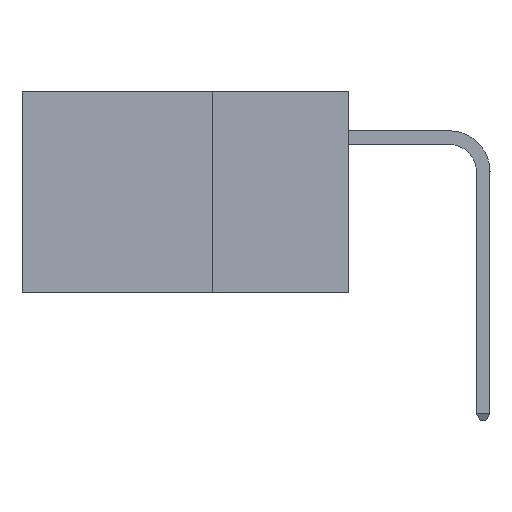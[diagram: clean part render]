
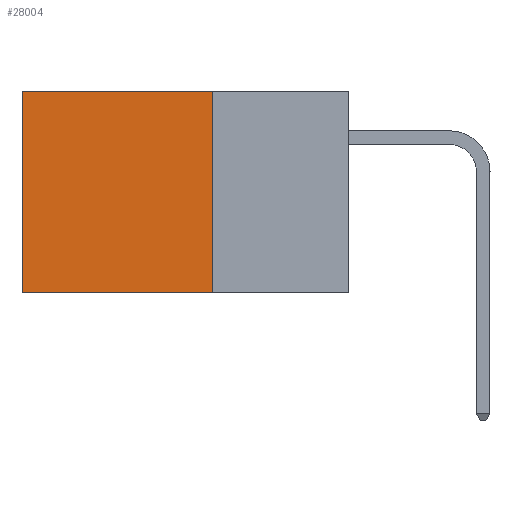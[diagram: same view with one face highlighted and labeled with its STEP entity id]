
A CAD part, left-side view. The second image highlights one B-rep face of the part: STEP entity #28004.
In plain terms, the highlighted planar face has unit normal (-1, 0, 0).
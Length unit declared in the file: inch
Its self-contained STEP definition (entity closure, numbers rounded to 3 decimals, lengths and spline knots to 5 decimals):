
#603 = ORIENTED_EDGE ( 'NONE', *, *, #15684, .F. ) ;
#860 = VERTEX_POINT ( 'NONE', #35887 ) ;
#2927 = LINE ( 'NONE', #18201, #37052 ) ;
#5528 = ORIENTED_EDGE ( 'NONE', *, *, #20811, .F. ) ;
#6387 = CARTESIAN_POINT ( 'NONE',  ( 0.2875, 0.25, 0. ) ) ;
#8119 = DIRECTION ( 'NONE',  ( 0., 1., 0. ) ) ;
#9584 = DIRECTION ( 'NONE',  ( 1., 0., 0. ) ) ;
#12715 = VERTEX_POINT ( 'NONE', #15642 ) ;
#13470 = VECTOR ( 'NONE', #40468, 39.37008 ) ;
#15327 = VERTEX_POINT ( 'NONE', #19901 ) ;
#15642 = CARTESIAN_POINT ( 'NONE',  ( 0.2875, 0.25, -0.37 ) ) ;
#15684 = EDGE_CURVE ( 'NONE', #22891, #12715, #33842, .T. ) ;
#16688 = CARTESIAN_POINT ( 'NONE',  ( 0.2875, 0.25, 0. ) ) ;
#17185 = DIRECTION ( 'NONE',  ( 0., 0., -1. ) ) ;
#17332 = CARTESIAN_POINT ( 'NONE',  ( 0.2875, 0.25, 0. ) ) ;
#18041 = ORIENTED_EDGE ( 'NONE', *, *, #27161, .T. ) ;
#18201 = CARTESIAN_POINT ( 'NONE',  ( 0.2875, 0.25, -0.37 ) ) ;
#19901 = CARTESIAN_POINT ( 'NONE',  ( 0.2875, 0.6, -0.37 ) ) ;
#20130 = AXIS2_PLACEMENT_3D ( 'NONE', #6387, #9584, #26041 ) ;
#20656 = CARTESIAN_POINT ( 'NONE',  ( 0.2875, 0.6, 0. ) ) ;
#20811 = EDGE_CURVE ( 'NONE', #12715, #15327, #2927, .T. ) ;
#21088 = FACE_OUTER_BOUND ( 'NONE', #32491, .T. ) ;
#22891 = VERTEX_POINT ( 'NONE', #16688 ) ;
#26041 = DIRECTION ( 'NONE',  ( 0., 0., -1. ) ) ;
#26178 = PLANE ( 'NONE',  #20130 ) ;
#27161 = EDGE_CURVE ( 'NONE', #22891, #860, #38223, .T. ) ;
#28004 = ADVANCED_FACE ( 'NONE', ( #21088 ), #26178, .F. ) ;
#30943 = LINE ( 'NONE', #20656, #35553 ) ;
#32491 = EDGE_LOOP ( 'NONE', ( #37121, #5528, #603, #18041 ) ) ;
#32589 = DIRECTION ( 'NONE',  ( 0., 0., -1. ) ) ;
#33842 = LINE ( 'NONE', #38629, #40558 ) ;
#35553 = VECTOR ( 'NONE', #17185, 39.37008 ) ;
#35887 = CARTESIAN_POINT ( 'NONE',  ( 0.2875, 0.6, 0. ) ) ;
#37052 = VECTOR ( 'NONE', #8119, 39.37008 ) ;
#37121 = ORIENTED_EDGE ( 'NONE', *, *, #40555, .T. ) ;
#38223 = LINE ( 'NONE', #17332, #13470 ) ;
#38629 = CARTESIAN_POINT ( 'NONE',  ( 0.2875, 0.25, 0. ) ) ;
#40468 = DIRECTION ( 'NONE',  ( 0., 1., 0. ) ) ;
#40555 = EDGE_CURVE ( 'NONE', #860, #15327, #30943, .T. ) ;
#40558 = VECTOR ( 'NONE', #32589, 39.37008 ) ;
